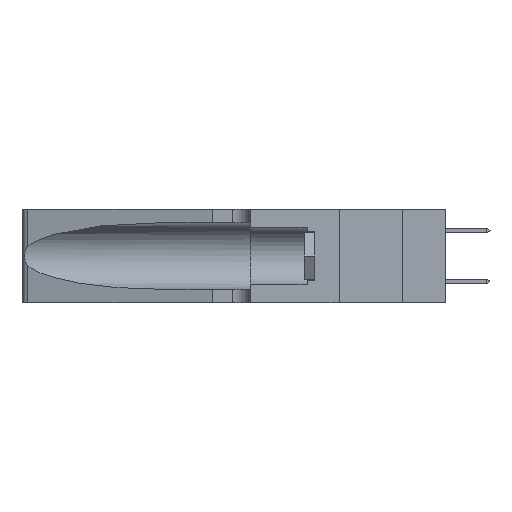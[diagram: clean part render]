
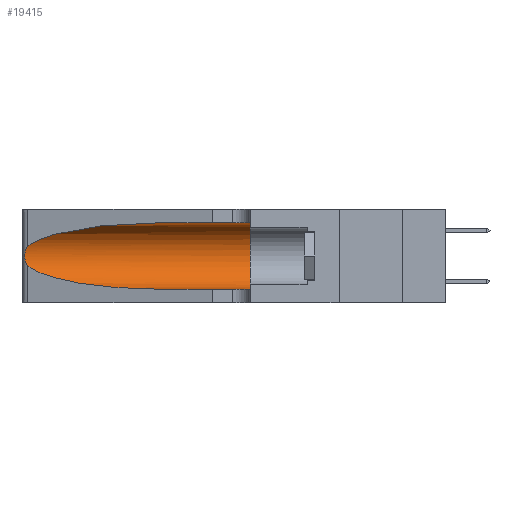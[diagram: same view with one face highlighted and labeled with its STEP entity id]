
A CAD part, left-side view. The second image highlights one B-rep face of the part: STEP entity #19415.
In plain terms, the highlighted cylindrical face has radius 3.308 mm (diameter 6.617 mm), a partial arc.
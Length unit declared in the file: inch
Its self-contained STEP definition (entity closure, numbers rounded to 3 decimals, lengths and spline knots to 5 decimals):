
#143 = VERTEX_POINT ( 'NONE', #19741 ) ;
#486 = VECTOR ( 'NONE', #10324, 39.37008 ) ;
#1579 = CARTESIAN_POINT ( 'NONE',  ( 0.25639, 1.23186, 0.15144 ) ) ;
#1731 = CARTESIAN_POINT ( 'NONE',  ( 0.1305, 0.72297, 0.31525 ) ) ;
#1909 = CARTESIAN_POINT ( 'NONE',  ( 0.25555, 1.22994, 0.2215 ) ) ;
#2210 = CARTESIAN_POINT ( 'NONE',  ( 0.1305, 0.72297, 0.31525 ) ) ;
#3007 = ORIENTED_EDGE ( 'NONE', *, *, #20614, .T. ) ;
#3083 = CARTESIAN_POINT ( 'NONE',  ( 0.25487, 1.22718, 0.22369 ) ) ;
#3557 = CIRCLE ( 'NONE', #14574, 0.13025 ) ;
#3700 = CARTESIAN_POINT ( 'NONE',  ( 0.26017, 1.23833, 0.17102 ) ) ;
#3996 = CARTESIAN_POINT ( 'NONE',  ( 0.25487, 1.22718, 0.14631 ) ) ;
#4273 = CARTESIAN_POINT ( 'NONE',  ( 0.1305, 0.35, 0.31525 ) ) ;
#4321 =( BOUNDED_CURVE ( )  B_SPLINE_CURVE ( 3, ( #2210, #16673, #21582, #15710 ),
 .UNSPECIFIED., .F., .F. ) 
 B_SPLINE_CURVE_WITH_KNOTS ( ( 4, 4 ),
 ( 1.5708, 2.84003 ),
 .UNSPECIFIED. ) 
 CURVE ( )  GEOMETRIC_REPRESENTATION_ITEM ( )  RATIONAL_B_SPLINE_CURVE ( ( 1., 0.87, 0.87, 1. ) ) 
 REPRESENTATION_ITEM ( '' )  );
#4455 = ORIENTED_EDGE ( 'NONE', *, *, #7770, .T. ) ;
#4702 = DIRECTION ( 'NONE',  ( 0., 0., 1. ) ) ;
#4976 = CARTESIAN_POINT ( 'NONE',  ( 0.1305, 0.35, 0.185 ) ) ;
#5402 = CARTESIAN_POINT ( 'NONE',  ( 0.1305, 0.72297, 0.05475 ) ) ;
#5656 = CARTESIAN_POINT ( 'NONE',  ( 0.25854, 1.2359, 0.20912 ) ) ;
#6026 = VERTEX_POINT ( 'NONE', #8034 ) ;
#6265 = LINE ( 'NONE', #26155, #486 ) ;
#6513 = CARTESIAN_POINT ( 'NONE',  ( 0.1305, 1.61858, 0.31525 ) ) ;
#7186 = VERTEX_POINT ( 'NONE', #4273 ) ;
#7770 = EDGE_CURVE ( 'NONE', #143, #6026, #6265, .T. ) ;
#7785 = DIRECTION ( 'NONE',  ( 0., 0., -1. ) ) ;
#7822 = VERTEX_POINT ( 'NONE', #3996 ) ;
#7833 = CARTESIAN_POINT ( 'NONE',  ( 0.26018, 1.23835, 0.19895 ) ) ;
#8034 = CARTESIAN_POINT ( 'NONE',  ( 0.1305, 0.35, 0.05475 ) ) ;
#8068 = CYLINDRICAL_SURFACE ( 'NONE', #22393, 0.13025 ) ;
#8832 = DIRECTION ( 'NONE',  ( 0., 1., 0. ) ) ;
#9241 = ORIENTED_EDGE ( 'NONE', *, *, #19156, .T. ) ;
#9287 = ORIENTED_EDGE ( 'NONE', *, *, #9616, .T. ) ;
#9616 = EDGE_CURVE ( 'NONE', #18139, #19047, #4321, .T. ) ;
#9753 = DIRECTION ( 'NONE',  ( 0., -1., 0. ) ) ;
#9959 = CARTESIAN_POINT ( 'NONE',  ( 0.25856, 1.23593, 0.16098 ) ) ;
#10324 = DIRECTION ( 'NONE',  ( 0., -1., 0. ) ) ;
#11995 = CARTESIAN_POINT ( 'NONE',  ( 0.25639, 1.23184, 0.21858 ) ) ;
#12495 =( BOUNDED_CURVE ( )  B_SPLINE_CURVE ( 3, ( #13735, #17529, #19598, #5402 ),
 .UNSPECIFIED., .F., .F. ) 
 B_SPLINE_CURVE_WITH_KNOTS ( ( 4, 4 ),
 ( 3.44316, 4.71239 ),
 .UNSPECIFIED. ) 
 CURVE ( )  GEOMETRIC_REPRESENTATION_ITEM ( )  RATIONAL_B_SPLINE_CURVE ( ( 1., 0.87, 0.87, 1. ) ) 
 REPRESENTATION_ITEM ( '' )  );
#12678 = EDGE_CURVE ( 'NONE', #7186, #6026, #3557, .T. ) ;
#13729 = CARTESIAN_POINT ( 'NONE',  ( 0.25555, 1.22993, 0.14849 ) ) ;
#13735 = CARTESIAN_POINT ( 'NONE',  ( 0.25487, 1.22718, 0.14631 ) ) ;
#14574 = AXIS2_PLACEMENT_3D ( 'NONE', #4976, #8832, #4702 ) ;
#15710 = CARTESIAN_POINT ( 'NONE',  ( 0.25487, 1.22718, 0.22369 ) ) ;
#16673 = CARTESIAN_POINT ( 'NONE',  ( 0.18966, 0.96281, 0.31525 ) ) ;
#17529 = CARTESIAN_POINT ( 'NONE',  ( 0.2373, 1.15595, 0.08982 ) ) ;
#17954 = VECTOR ( 'NONE', #22411, 39.37008 ) ;
#17976 = CARTESIAN_POINT ( 'NONE',  ( 0.26075, 1.23896, 0.19203 ) ) ;
#18139 = VERTEX_POINT ( 'NONE', #1731 ) ;
#19047 = VERTEX_POINT ( 'NONE', #3083 ) ;
#19156 = EDGE_CURVE ( 'NONE', #7822, #143, #12495, .T. ) ;
#19415 = ADVANCED_FACE ( 'NONE', ( #21381 ), #8068, .F. ) ;
#19540 = EDGE_LOOP ( 'NONE', ( #9287, #3007, #9241, #4455, #21601, #25801 ) ) ;
#19598 = CARTESIAN_POINT ( 'NONE',  ( 0.18966, 0.96281, 0.05475 ) ) ;
#19741 = CARTESIAN_POINT ( 'NONE',  ( 0.1305, 0.72297, 0.05475 ) ) ;
#19867 = CARTESIAN_POINT ( 'NONE',  ( 0.25787, 1.23484, 0.2124 ) ) ;
#20033 = CARTESIAN_POINT ( 'NONE',  ( 0.26075, 1.23896, 0.178 ) ) ;
#20209 = CARTESIAN_POINT ( 'NONE',  ( 0.25789, 1.23486, 0.15765 ) ) ;
#20614 = EDGE_CURVE ( 'NONE', #19047, #7822, #25959, .T. ) ;
#21381 = FACE_OUTER_BOUND ( 'NONE', #19540, .T. ) ;
#21582 = CARTESIAN_POINT ( 'NONE',  ( 0.2373, 1.15595, 0.28018 ) ) ;
#21601 = ORIENTED_EDGE ( 'NONE', *, *, #12678, .F. ) ;
#22393 = AXIS2_PLACEMENT_3D ( 'NONE', #23779, #9753, #7785 ) ;
#22411 = DIRECTION ( 'NONE',  ( 0., -1., 0. ) ) ;
#22705 = LINE ( 'NONE', #6513, #17954 ) ;
#23779 = CARTESIAN_POINT ( 'NONE',  ( 0.1305, 1.61858, 0.185 ) ) ;
#23867 = EDGE_CURVE ( 'NONE', #18139, #7186, #22705, .T. ) ;
#25801 = ORIENTED_EDGE ( 'NONE', *, *, #23867, .F. ) ;
#25959 = B_SPLINE_CURVE_WITH_KNOTS ( 'NONE', 3,
 ( #26025, #1909, #11995, #19867, #5656, #7833, #17976, #20033, #3700, #9959, #20209, #1579, #13729, #26114 ),
 .UNSPECIFIED., .F., .F.,
 ( 4, 2, 2, 2, 2, 2, 4 ),
 ( 0., 0.00027, 0.00053, 0.00107, 0.0016, 0.00187, 0.00214 ),
 .UNSPECIFIED. ) ;
#26025 = CARTESIAN_POINT ( 'NONE',  ( 0.25487, 1.22718, 0.22369 ) ) ;
#26114 = CARTESIAN_POINT ( 'NONE',  ( 0.25487, 1.22718, 0.14631 ) ) ;
#26155 = CARTESIAN_POINT ( 'NONE',  ( 0.1305, 1.61858, 0.05475 ) ) ;
